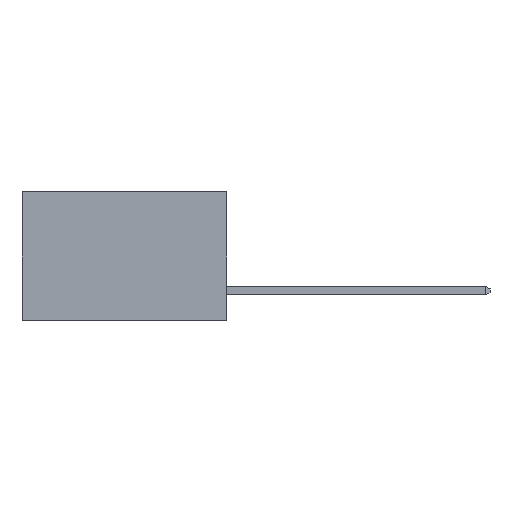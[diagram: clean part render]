
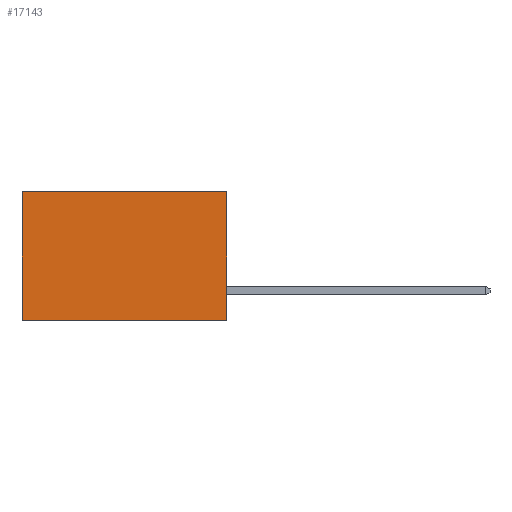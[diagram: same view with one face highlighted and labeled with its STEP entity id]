
A CAD part, left-side view. The second image highlights one B-rep face of the part: STEP entity #17143.
In plain terms, the highlighted planar face has unit normal (-1, 0, 0).
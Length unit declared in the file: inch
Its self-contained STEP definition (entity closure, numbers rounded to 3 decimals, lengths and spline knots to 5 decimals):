
#999 = ORIENTED_EDGE ( 'NONE', *, *, #25992, .F. ) ;
#1092 = DIRECTION ( 'NONE',  ( 0., 1., 0. ) ) ;
#2699 = DIRECTION ( 'NONE',  ( 0., 0., -1. ) ) ;
#3158 = LINE ( 'NONE', #6689, #20885 ) ;
#6689 = CARTESIAN_POINT ( 'NONE',  ( 0.277, 0.59, -0.37 ) ) ;
#7515 = VERTEX_POINT ( 'NONE', #27651 ) ;
#7975 = VERTEX_POINT ( 'NONE', #19028 ) ;
#7980 = ORIENTED_EDGE ( 'NONE', *, *, #22566, .F. ) ;
#8150 = EDGE_LOOP ( 'NONE', ( #8805, #999, #7980, #18795 ) ) ;
#8805 = ORIENTED_EDGE ( 'NONE', *, *, #11233, .T. ) ;
#11189 = VECTOR ( 'NONE', #23746, 39.37008 ) ;
#11233 = EDGE_CURVE ( 'NONE', #7975, #11262, #3158, .T. ) ;
#11262 = VERTEX_POINT ( 'NONE', #24369 ) ;
#11604 = FACE_OUTER_BOUND ( 'NONE', #8150, .T. ) ;
#11641 = PLANE ( 'NONE',  #28494 ) ;
#12680 = LINE ( 'NONE', #12694, #23977 ) ;
#12694 = CARTESIAN_POINT ( 'NONE',  ( 0.277, 0., -0.37 ) ) ;
#13507 = LINE ( 'NONE', #21130, #25119 ) ;
#14024 = VERTEX_POINT ( 'NONE', #24276 ) ;
#15563 = DIRECTION ( 'NONE',  ( 0., 0., -1. ) ) ;
#16051 = DIRECTION ( 'NONE',  ( 1., 0., 0. ) ) ;
#17143 = ADVANCED_FACE ( 'NONE', ( #11604 ), #11641, .F. ) ;
#18157 = EDGE_CURVE ( 'NONE', #14024, #7975, #28616, .T. ) ;
#18795 = ORIENTED_EDGE ( 'NONE', *, *, #18157, .T. ) ;
#19028 = CARTESIAN_POINT ( 'NONE',  ( 0.277, 0.59, 0. ) ) ;
#20885 = VECTOR ( 'NONE', #15563, 39.37008 ) ;
#21130 = CARTESIAN_POINT ( 'NONE',  ( 0.277, 0., -0.37 ) ) ;
#22566 = EDGE_CURVE ( 'NONE', #14024, #7515, #12680, .T. ) ;
#23746 = DIRECTION ( 'NONE',  ( 0., 1., 0. ) ) ;
#23977 = VECTOR ( 'NONE', #25746, 39.37008 ) ;
#24276 = CARTESIAN_POINT ( 'NONE',  ( 0.277, 0., 0. ) ) ;
#24369 = CARTESIAN_POINT ( 'NONE',  ( 0.277, 0.59, -0.37 ) ) ;
#25119 = VECTOR ( 'NONE', #1092, 39.37008 ) ;
#25746 = DIRECTION ( 'NONE',  ( 0., 0., -1. ) ) ;
#25914 = CARTESIAN_POINT ( 'NONE',  ( 0.277, 0., 0. ) ) ;
#25992 = EDGE_CURVE ( 'NONE', #7515, #11262, #13507, .T. ) ;
#26894 = CARTESIAN_POINT ( 'NONE',  ( 0.277, 0., -0.37 ) ) ;
#27651 = CARTESIAN_POINT ( 'NONE',  ( 0.277, 0., -0.37 ) ) ;
#28494 = AXIS2_PLACEMENT_3D ( 'NONE', #26894, #16051, #2699 ) ;
#28616 = LINE ( 'NONE', #25914, #11189 ) ;
